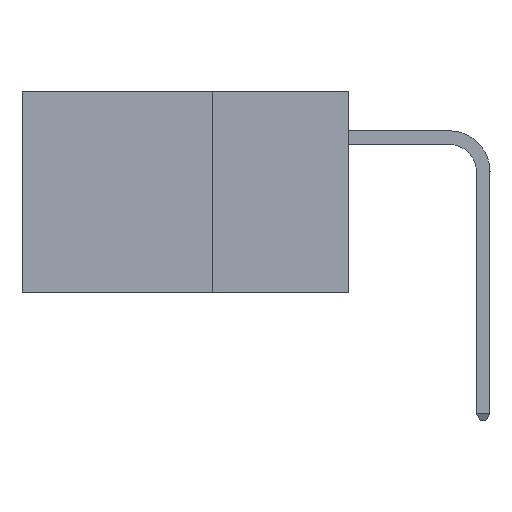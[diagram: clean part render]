
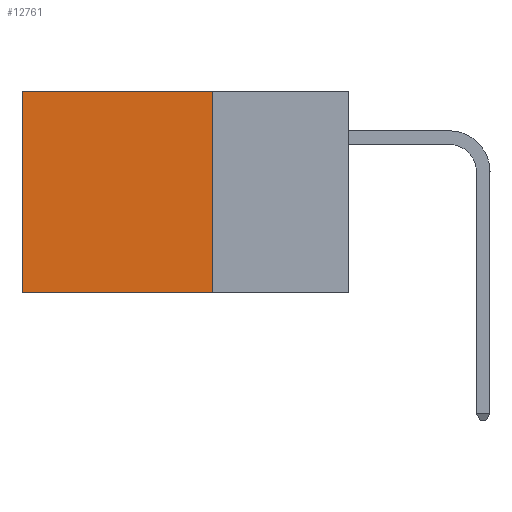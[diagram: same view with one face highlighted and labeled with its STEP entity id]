
A CAD part, left-side view. The second image highlights one B-rep face of the part: STEP entity #12761.
In plain terms, the highlighted planar face has unit normal (-1, 0, 0).
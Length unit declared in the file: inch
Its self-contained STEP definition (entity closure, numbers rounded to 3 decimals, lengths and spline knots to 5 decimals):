
#25 = CARTESIAN_POINT ( 'NONE',  ( 0.2875, 0.6, 0. ) ) ;
#809 = EDGE_LOOP ( 'NONE', ( #1980, #3679, #3102, #13128 ) ) ;
#1065 = EDGE_CURVE ( 'NONE', #10466, #11426, #21628, .T. ) ;
#1980 = ORIENTED_EDGE ( 'NONE', *, *, #1065, .T. ) ;
#2996 = VECTOR ( 'NONE', #3681, 39.37008 ) ;
#3102 = ORIENTED_EDGE ( 'NONE', *, *, #14249, .F. ) ;
#3403 = VECTOR ( 'NONE', #12673, 39.37008 ) ;
#3679 = ORIENTED_EDGE ( 'NONE', *, *, #14849, .F. ) ;
#3681 = DIRECTION ( 'NONE',  ( 0., 1., 0. ) ) ;
#3720 = LINE ( 'NONE', #10260, #2996 ) ;
#4544 = CARTESIAN_POINT ( 'NONE',  ( 0.2875, 0.25, -0.37 ) ) ;
#4913 = VERTEX_POINT ( 'NONE', #20255 ) ;
#7270 = CARTESIAN_POINT ( 'NONE',  ( 0.2875, 0.25, 0. ) ) ;
#8087 = VECTOR ( 'NONE', #12715, 39.37008 ) ;
#8244 = DIRECTION ( 'NONE',  ( 0., 0., -1. ) ) ;
#9472 = DIRECTION ( 'NONE',  ( 0., 0., -1. ) ) ;
#9546 = VERTEX_POINT ( 'NONE', #4544 ) ;
#9667 = VECTOR ( 'NONE', #8244, 39.37008 ) ;
#9981 = EDGE_CURVE ( 'NONE', #4913, #10466, #14511, .T. ) ;
#10260 = CARTESIAN_POINT ( 'NONE',  ( 0.2875, 0.25, -0.37 ) ) ;
#10466 = VERTEX_POINT ( 'NONE', #22945 ) ;
#11426 = VERTEX_POINT ( 'NONE', #26539 ) ;
#12673 = DIRECTION ( 'NONE',  ( 0., 0., -1. ) ) ;
#12715 = DIRECTION ( 'NONE',  ( 0., 1., 0. ) ) ;
#12761 = ADVANCED_FACE ( 'NONE', ( #19059 ), #15833, .F. ) ;
#13128 = ORIENTED_EDGE ( 'NONE', *, *, #9981, .T. ) ;
#14249 = EDGE_CURVE ( 'NONE', #4913, #9546, #14395, .T. ) ;
#14395 = LINE ( 'NONE', #27467, #3403 ) ;
#14511 = LINE ( 'NONE', #21075, #8087 ) ;
#14849 = EDGE_CURVE ( 'NONE', #9546, #11426, #3720, .T. ) ;
#15833 = PLANE ( 'NONE',  #26083 ) ;
#19059 = FACE_OUTER_BOUND ( 'NONE', #809, .T. ) ;
#20255 = CARTESIAN_POINT ( 'NONE',  ( 0.2875, 0.25, 0. ) ) ;
#21075 = CARTESIAN_POINT ( 'NONE',  ( 0.2875, 0.25, 0. ) ) ;
#21628 = LINE ( 'NONE', #25, #9667 ) ;
#22182 = DIRECTION ( 'NONE',  ( 1., 0., 0. ) ) ;
#22945 = CARTESIAN_POINT ( 'NONE',  ( 0.2875, 0.6, 0. ) ) ;
#26083 = AXIS2_PLACEMENT_3D ( 'NONE', #7270, #22182, #9472 ) ;
#26539 = CARTESIAN_POINT ( 'NONE',  ( 0.2875, 0.6, -0.37 ) ) ;
#27467 = CARTESIAN_POINT ( 'NONE',  ( 0.2875, 0.25, 0. ) ) ;
